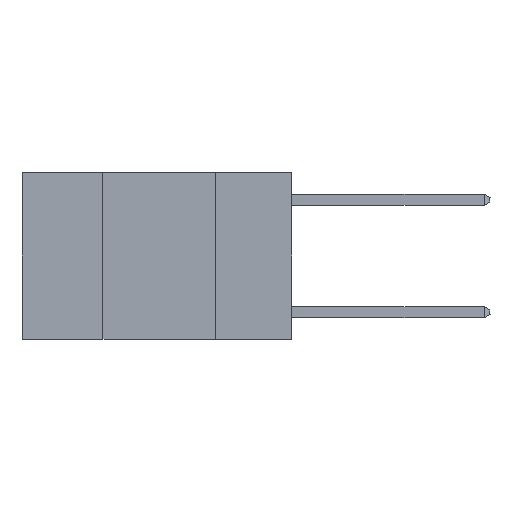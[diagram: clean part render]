
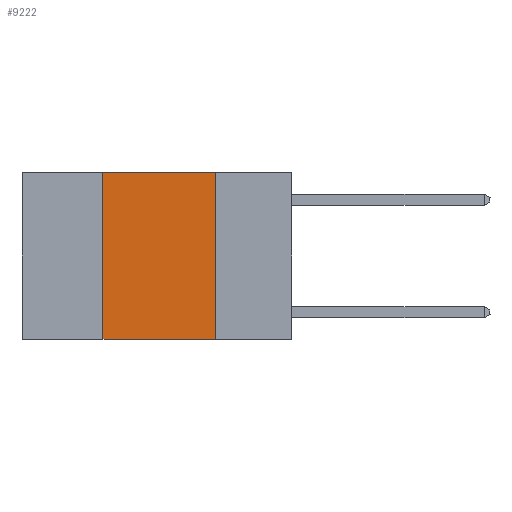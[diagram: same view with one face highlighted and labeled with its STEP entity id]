
A CAD part, left-side view. The second image highlights one B-rep face of the part: STEP entity #9222.
In plain terms, the highlighted planar face has unit normal (-1, 0, 0).
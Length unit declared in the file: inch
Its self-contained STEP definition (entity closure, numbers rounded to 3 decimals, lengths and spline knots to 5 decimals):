
#800 = CARTESIAN_POINT ( 'NONE',  ( 0., 0.42, 0. ) ) ;
#1271 = CARTESIAN_POINT ( 'NONE',  ( 0., 0.6, 0. ) ) ;
#1389 = ORIENTED_EDGE ( 'NONE', *, *, #13889, .F. ) ;
#2050 = DIRECTION ( 'NONE',  ( 0., -1., 0. ) ) ;
#3370 = DIRECTION ( 'NONE',  ( 0., 0., -1. ) ) ;
#4348 = DIRECTION ( 'NONE',  ( 0., 0., 1. ) ) ;
#4703 = VECTOR ( 'NONE', #3370, 39.37008 ) ;
#4943 = DIRECTION ( 'NONE',  ( 1., 0., 0. ) ) ;
#5045 = VERTEX_POINT ( 'NONE', #6147 ) ;
#6041 = VERTEX_POINT ( 'NONE', #8421 ) ;
#6147 = CARTESIAN_POINT ( 'NONE',  ( 0., 0.42, -0.37 ) ) ;
#6802 = EDGE_CURVE ( 'NONE', #5045, #6041, #10277, .T. ) ;
#6803 = CARTESIAN_POINT ( 'NONE',  ( 0., 0.17, -0.37 ) ) ;
#6930 = LINE ( 'NONE', #7080, #4703 ) ;
#7016 = VERTEX_POINT ( 'NONE', #10727 ) ;
#7080 = CARTESIAN_POINT ( 'NONE',  ( 0., 0.17, 0. ) ) ;
#7231 = EDGE_CURVE ( 'NONE', #5045, #12232, #10562, .T. ) ;
#7574 = DIRECTION ( 'NONE',  ( 0., 0., -1. ) ) ;
#8396 = LINE ( 'NONE', #12201, #9110 ) ;
#8421 = CARTESIAN_POINT ( 'NONE',  ( 0., 0.42, 0. ) ) ;
#9110 = VECTOR ( 'NONE', #12030, 39.37008 ) ;
#9222 = ADVANCED_FACE ( 'NONE', ( #13573 ), #12327, .F. ) ;
#9649 = VECTOR ( 'NONE', #4348, 39.37008 ) ;
#9761 = AXIS2_PLACEMENT_3D ( 'NONE', #1271, #4943, #7574 ) ;
#9823 = ORIENTED_EDGE ( 'NONE', *, *, #10555, .F. ) ;
#10168 = EDGE_LOOP ( 'NONE', ( #1389, #9823, #11669, #14164 ) ) ;
#10277 = LINE ( 'NONE', #800, #9649 ) ;
#10409 = CARTESIAN_POINT ( 'NONE',  ( 0., 0.6, -0.37 ) ) ;
#10555 = EDGE_CURVE ( 'NONE', #6041, #7016, #8396, .T. ) ;
#10562 = LINE ( 'NONE', #10409, #15463 ) ;
#10727 = CARTESIAN_POINT ( 'NONE',  ( 0., 0.17, 0. ) ) ;
#11669 = ORIENTED_EDGE ( 'NONE', *, *, #6802, .F. ) ;
#12030 = DIRECTION ( 'NONE',  ( 0., -1., 0. ) ) ;
#12201 = CARTESIAN_POINT ( 'NONE',  ( 0., 0.6, 0. ) ) ;
#12232 = VERTEX_POINT ( 'NONE', #6803 ) ;
#12327 = PLANE ( 'NONE',  #9761 ) ;
#13573 = FACE_OUTER_BOUND ( 'NONE', #10168, .T. ) ;
#13889 = EDGE_CURVE ( 'NONE', #7016, #12232, #6930, .T. ) ;
#14164 = ORIENTED_EDGE ( 'NONE', *, *, #7231, .T. ) ;
#15463 = VECTOR ( 'NONE', #2050, 39.37008 ) ;
